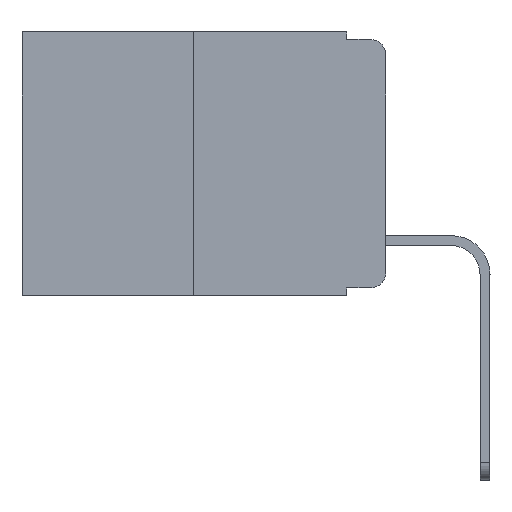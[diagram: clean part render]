
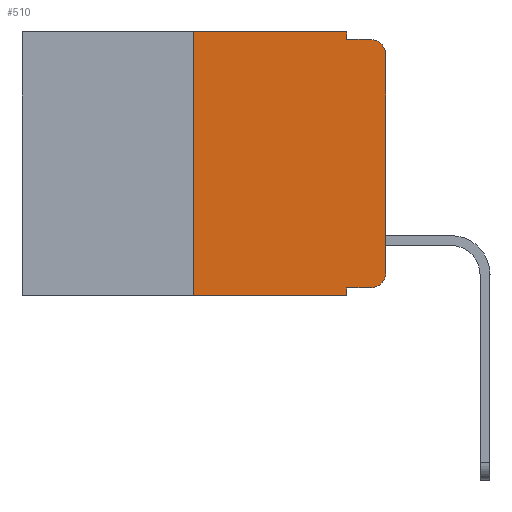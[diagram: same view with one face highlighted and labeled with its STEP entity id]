
A CAD part, left-side view. The second image highlights one B-rep face of the part: STEP entity #510.
In plain terms, the highlighted planar face has unit normal (-1, 0, 0).
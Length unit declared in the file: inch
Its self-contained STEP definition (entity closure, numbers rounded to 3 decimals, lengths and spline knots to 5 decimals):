
#211 = DIRECTION ( 'NONE',  ( 0., -1., 0. ) ) ;
#364 = CARTESIAN_POINT ( 'NONE',  ( 0., 0.25, -0.343 ) ) ;
#381 = FACE_OUTER_BOUND ( 'NONE', #8795, .T. ) ;
#510 = ADVANCED_FACE ( 'NONE', ( #381 ), #9043, .F. ) ;
#545 = ORIENTED_EDGE ( 'NONE', *, *, #11024, .T. ) ;
#635 = DIRECTION ( 'NONE',  ( 0., 0., 1. ) ) ;
#675 = LINE ( 'NONE', #11031, #5185 ) ;
#836 = CARTESIAN_POINT ( 'NONE',  ( 0., 0.02, -0.01 ) ) ;
#943 = ORIENTED_EDGE ( 'NONE', *, *, #6790, .F. ) ;
#1083 = ORIENTED_EDGE ( 'NONE', *, *, #6274, .F. ) ;
#1116 = DIRECTION ( 'NONE',  ( -1., 0., 0. ) ) ;
#1195 = CARTESIAN_POINT ( 'NONE',  ( 0., 0.051, -0.333 ) ) ;
#1532 = VERTEX_POINT ( 'NONE', #8268 ) ;
#1579 = AXIS2_PLACEMENT_3D ( 'NONE', #7180, #1744, #2694 ) ;
#1744 = DIRECTION ( 'NONE',  ( 1., 0., 0. ) ) ;
#1853 = DIRECTION ( 'NONE',  ( 0., -1., 0. ) ) ;
#2016 = VERTEX_POINT ( 'NONE', #11019 ) ;
#2130 = EDGE_CURVE ( 'NONE', #2016, #10024, #5119, .T. ) ;
#2133 = DIRECTION ( 'NONE',  ( 0., 0., -1. ) ) ;
#2403 = EDGE_CURVE ( 'NONE', #1532, #10024, #6210, .T. ) ;
#2626 = CARTESIAN_POINT ( 'NONE',  ( 0., 0.02, -0.313 ) ) ;
#2686 = CARTESIAN_POINT ( 'NONE',  ( 0., 0.473, -0.343 ) ) ;
#2694 = DIRECTION ( 'NONE',  ( 0., 0., -1. ) ) ;
#2703 = VERTEX_POINT ( 'NONE', #10075 ) ;
#2817 = VERTEX_POINT ( 'NONE', #3558 ) ;
#2847 = DIRECTION ( 'NONE',  ( 0., 0., -1. ) ) ;
#2905 = VECTOR ( 'NONE', #211, 39.37008 ) ;
#3414 = VECTOR ( 'NONE', #6916, 39.37008 ) ;
#3450 = DIRECTION ( 'NONE',  ( -1., 0., 0. ) ) ;
#3464 = CARTESIAN_POINT ( 'NONE',  ( 0., 0., -0.313 ) ) ;
#3558 = CARTESIAN_POINT ( 'NONE',  ( 0., 0.051, 0. ) ) ;
#3561 = LINE ( 'NONE', #5039, #8604 ) ;
#3734 = CARTESIAN_POINT ( 'NONE',  ( 0., 0.02, -0.03 ) ) ;
#4699 = CARTESIAN_POINT ( 'NONE',  ( 0., 0.051, -0.333 ) ) ;
#4868 = VECTOR ( 'NONE', #2133, 39.37008 ) ;
#5039 = CARTESIAN_POINT ( 'NONE',  ( 0., 0.25, 0. ) ) ;
#5119 = LINE ( 'NONE', #10284, #7609 ) ;
#5185 = VECTOR ( 'NONE', #5781, 39.37008 ) ;
#5509 = AXIS2_PLACEMENT_3D ( 'NONE', #2626, #3450, #8841 ) ;
#5525 = VERTEX_POINT ( 'NONE', #4699 ) ;
#5659 = ORIENTED_EDGE ( 'NONE', *, *, #8465, .F. ) ;
#5682 = LINE ( 'NONE', #9254, #9145 ) ;
#5781 = DIRECTION ( 'NONE',  ( 0., 0., -1. ) ) ;
#5990 = CARTESIAN_POINT ( 'NONE',  ( 0., 0.473, 0. ) ) ;
#6210 = CIRCLE ( 'NONE', #7888, 0.02 ) ;
#6274 = EDGE_CURVE ( 'NONE', #2817, #2016, #675, .T. ) ;
#6470 = ORIENTED_EDGE ( 'NONE', *, *, #2130, .F. ) ;
#6790 = EDGE_CURVE ( 'NONE', #5525, #6852, #8345, .T. ) ;
#6810 = VECTOR ( 'NONE', #1853, 39.37008 ) ;
#6852 = VERTEX_POINT ( 'NONE', #7351 ) ;
#6916 = DIRECTION ( 'NONE',  ( 0., -1., 0. ) ) ;
#7180 = CARTESIAN_POINT ( 'NONE',  ( 0., 0.473, 0. ) ) ;
#7333 = EDGE_CURVE ( 'NONE', #9345, #6852, #9168, .T. ) ;
#7351 = CARTESIAN_POINT ( 'NONE',  ( 0., 0.051, -0.343 ) ) ;
#7588 = ORIENTED_EDGE ( 'NONE', *, *, #9553, .T. ) ;
#7609 = VECTOR ( 'NONE', #9435, 39.37008 ) ;
#7770 = EDGE_CURVE ( 'NONE', #9345, #2703, #3561, .T. ) ;
#7888 = AXIS2_PLACEMENT_3D ( 'NONE', #3734, #1116, #2847 ) ;
#8082 = ORIENTED_EDGE ( 'NONE', *, *, #2403, .T. ) ;
#8161 = EDGE_CURVE ( 'NONE', #10804, #1532, #5682, .T. ) ;
#8268 = CARTESIAN_POINT ( 'NONE',  ( 0., 0., -0.03 ) ) ;
#8318 = CARTESIAN_POINT ( 'NONE',  ( 0., 0.051, 0. ) ) ;
#8338 = LINE ( 'NONE', #1195, #2905 ) ;
#8345 = LINE ( 'NONE', #8318, #4868 ) ;
#8465 = EDGE_CURVE ( 'NONE', #2703, #2817, #11498, .T. ) ;
#8604 = VECTOR ( 'NONE', #635, 39.37008 ) ;
#8795 = EDGE_LOOP ( 'NONE', ( #11272, #8082, #6470, #1083, #5659, #10174, #10327, #943, #545, #7588 ) ) ;
#8841 = DIRECTION ( 'NONE',  ( 0., 0., -1. ) ) ;
#9043 = PLANE ( 'NONE',  #1579 ) ;
#9095 = CARTESIAN_POINT ( 'NONE',  ( 0., 0.02, -0.333 ) ) ;
#9145 = VECTOR ( 'NONE', #11069, 39.37008 ) ;
#9168 = LINE ( 'NONE', #2686, #6810 ) ;
#9254 = CARTESIAN_POINT ( 'NONE',  ( 0., 0., 0. ) ) ;
#9345 = VERTEX_POINT ( 'NONE', #364 ) ;
#9435 = DIRECTION ( 'NONE',  ( 0., -1., 0. ) ) ;
#9553 = EDGE_CURVE ( 'NONE', #10385, #10804, #11066, .T. ) ;
#10024 = VERTEX_POINT ( 'NONE', #836 ) ;
#10075 = CARTESIAN_POINT ( 'NONE',  ( 0., 0.25, 0. ) ) ;
#10174 = ORIENTED_EDGE ( 'NONE', *, *, #7770, .F. ) ;
#10284 = CARTESIAN_POINT ( 'NONE',  ( 0., 0.051, -0.01 ) ) ;
#10327 = ORIENTED_EDGE ( 'NONE', *, *, #7333, .T. ) ;
#10385 = VERTEX_POINT ( 'NONE', #9095 ) ;
#10804 = VERTEX_POINT ( 'NONE', #3464 ) ;
#11019 = CARTESIAN_POINT ( 'NONE',  ( 0., 0.051, -0.01 ) ) ;
#11024 = EDGE_CURVE ( 'NONE', #5525, #10385, #8338, .T. ) ;
#11031 = CARTESIAN_POINT ( 'NONE',  ( 0., 0.051, 0. ) ) ;
#11066 = CIRCLE ( 'NONE', #5509, 0.02 ) ;
#11069 = DIRECTION ( 'NONE',  ( 0., 0., 1. ) ) ;
#11272 = ORIENTED_EDGE ( 'NONE', *, *, #8161, .T. ) ;
#11498 = LINE ( 'NONE', #5990, #3414 ) ;
